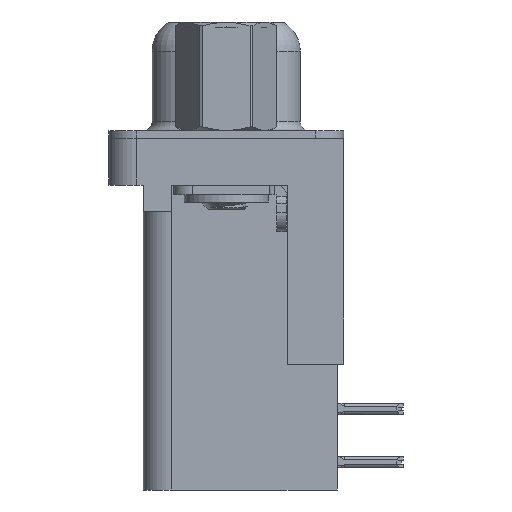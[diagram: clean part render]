
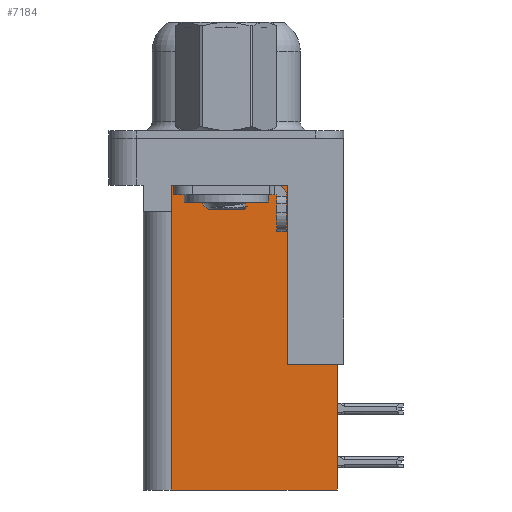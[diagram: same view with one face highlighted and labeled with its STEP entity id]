
A CAD part, left-side view. The second image highlights one B-rep face of the part: STEP entity #7184.
In plain terms, the highlighted planar face has unit normal (-1, 0, 0).
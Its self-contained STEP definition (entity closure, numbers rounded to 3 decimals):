
#81 = CARTESIAN_POINT ( 'NONE',  ( 3.79, 2.925, -18.76 ) ) ;
#88 = VECTOR ( 'NONE', #13437, 1000. ) ;
#1616 = CARTESIAN_POINT ( 'NONE',  ( 3.79, -3.295, -18.76 ) ) ;
#1933 = VECTOR ( 'NONE', #28730, 1000. ) ;
#2948 = LINE ( 'NONE', #13795, #8123 ) ;
#3686 = VECTOR ( 'NONE', #10460, 1000. ) ;
#3858 = ORIENTED_EDGE ( 'NONE', *, *, #18213, .F. ) ;
#5352 = CARTESIAN_POINT ( 'NONE',  ( 3.79, -3.295, -18.76 ) ) ;
#5602 = ORIENTED_EDGE ( 'NONE', *, *, #17219, .F. ) ;
#6007 = CARTESIAN_POINT ( 'NONE',  ( 3.79, 2.925, -18.76 ) ) ;
#7184 = ADVANCED_FACE ( 'NONE', ( #8593 ), #12050, .F. ) ;
#8123 = VECTOR ( 'NONE', #16025, 1000. ) ;
#8344 = EDGE_CURVE ( 'NONE', #25101, #24988, #26606, .T. ) ;
#8593 = FACE_OUTER_BOUND ( 'NONE', #12820, .T. ) ;
#9993 = EDGE_CURVE ( 'NONE', #13525, #28580, #10281, .T. ) ;
#10281 = LINE ( 'NONE', #16833, #27269 ) ;
#10460 = DIRECTION ( 'NONE',  ( 0., 0., 1. ) ) ;
#11072 = EDGE_CURVE ( 'NONE', #17729, #12175, #26557, .T. ) ;
#11920 = ORIENTED_EDGE ( 'NONE', *, *, #8344, .T. ) ;
#11925 = LINE ( 'NONE', #24490, #88 ) ;
#12050 = PLANE ( 'NONE',  #18261 ) ;
#12175 = VERTEX_POINT ( 'NONE', #27775 ) ;
#12354 = DIRECTION ( 'NONE',  ( 0., 0., -1. ) ) ;
#12820 = EDGE_LOOP ( 'NONE', ( #28419, #23403, #11920, #3858, #5602, #22418, #13931, #23066 ) ) ;
#13437 = DIRECTION ( 'NONE',  ( 0., 1., 0. ) ) ;
#13525 = VERTEX_POINT ( 'NONE', #14794 ) ;
#13600 = CARTESIAN_POINT ( 'NONE',  ( 3.79, 0., -3.9 ) ) ;
#13795 = CARTESIAN_POINT ( 'NONE',  ( 3.79, 2.895, -3.9 ) ) ;
#13931 = ORIENTED_EDGE ( 'NONE', *, *, #15294, .T. ) ;
#14100 = VECTOR ( 'NONE', #20130, 1000. ) ;
#14294 = DIRECTION ( 'NONE',  ( 0., 1., 0. ) ) ;
#14794 = CARTESIAN_POINT ( 'NONE',  ( 3.79, -5.925, -12.05 ) ) ;
#14895 = CARTESIAN_POINT ( 'NONE',  ( 3.79, 2.895, -2.5 ) ) ;
#15294 = EDGE_CURVE ( 'NONE', #13525, #17729, #24818, .T. ) ;
#16011 = VERTEX_POINT ( 'NONE', #14895 ) ;
#16025 = DIRECTION ( 'NONE',  ( 0., 0., -1. ) ) ;
#16328 = EDGE_CURVE ( 'NONE', #16011, #25101, #2948, .T. ) ;
#16833 = CARTESIAN_POINT ( 'NONE',  ( 3.79, -5.925, -2. ) ) ;
#17219 = EDGE_CURVE ( 'NONE', #28580, #28589, #11925, .T. ) ;
#17436 = LINE ( 'NONE', #6007, #23364 ) ;
#17729 = VERTEX_POINT ( 'NONE', #26688 ) ;
#18213 = EDGE_CURVE ( 'NONE', #28589, #24988, #17436, .T. ) ;
#18261 = AXIS2_PLACEMENT_3D ( 'NONE', #5352, #27570, #14294 ) ;
#19977 = LINE ( 'NONE', #20035, #14100 ) ;
#19995 = CARTESIAN_POINT ( 'NONE',  ( 3.79, -5.925, -18.76 ) ) ;
#20035 = CARTESIAN_POINT ( 'NONE',  ( 3.79, -3.295, -2.5 ) ) ;
#20130 = DIRECTION ( 'NONE',  ( 0., 1., 0. ) ) ;
#20728 = VECTOR ( 'NONE', #22530, 1000. ) ;
#20787 = EDGE_CURVE ( 'NONE', #12175, #16011, #19977, .T. ) ;
#21548 = DIRECTION ( 'NONE',  ( 0., 0., 1. ) ) ;
#22418 = ORIENTED_EDGE ( 'NONE', *, *, #9993, .F. ) ;
#22530 = DIRECTION ( 'NONE',  ( 0., 1., 0. ) ) ;
#23066 = ORIENTED_EDGE ( 'NONE', *, *, #11072, .T. ) ;
#23364 = VECTOR ( 'NONE', #21548, 1000. ) ;
#23403 = ORIENTED_EDGE ( 'NONE', *, *, #16328, .T. ) ;
#24490 = CARTESIAN_POINT ( 'NONE',  ( 3.79, -3.295, -18.76 ) ) ;
#24659 = CARTESIAN_POINT ( 'NONE',  ( 3.79, 2.925, -3.9 ) ) ;
#24818 = LINE ( 'NONE', #28636, #1933 ) ;
#24988 = VERTEX_POINT ( 'NONE', #24659 ) ;
#25101 = VERTEX_POINT ( 'NONE', #25934 ) ;
#25934 = CARTESIAN_POINT ( 'NONE',  ( 3.79, 2.895, -3.9 ) ) ;
#26557 = LINE ( 'NONE', #1616, #3686 ) ;
#26606 = LINE ( 'NONE', #13600, #20728 ) ;
#26688 = CARTESIAN_POINT ( 'NONE',  ( 3.79, -3.295, -12.05 ) ) ;
#27269 = VECTOR ( 'NONE', #12354, 1000. ) ;
#27570 = DIRECTION ( 'NONE',  ( 1., 0., 0. ) ) ;
#27775 = CARTESIAN_POINT ( 'NONE',  ( 3.79, -3.295, -2.5 ) ) ;
#28419 = ORIENTED_EDGE ( 'NONE', *, *, #20787, .T. ) ;
#28580 = VERTEX_POINT ( 'NONE', #19995 ) ;
#28589 = VERTEX_POINT ( 'NONE', #81 ) ;
#28636 = CARTESIAN_POINT ( 'NONE',  ( 3.79, -6.295, -12.05 ) ) ;
#28730 = DIRECTION ( 'NONE',  ( 0., 1., 0. ) ) ;
